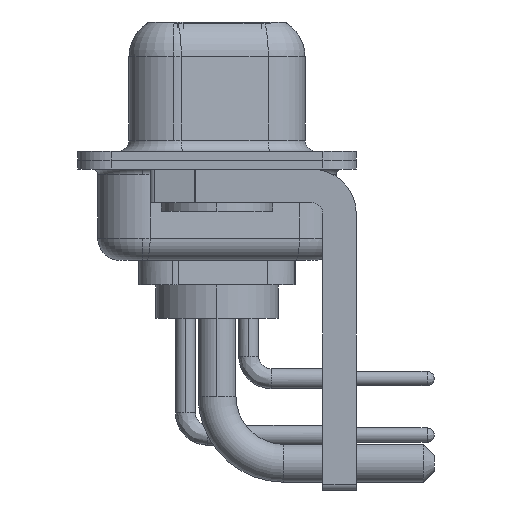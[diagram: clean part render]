
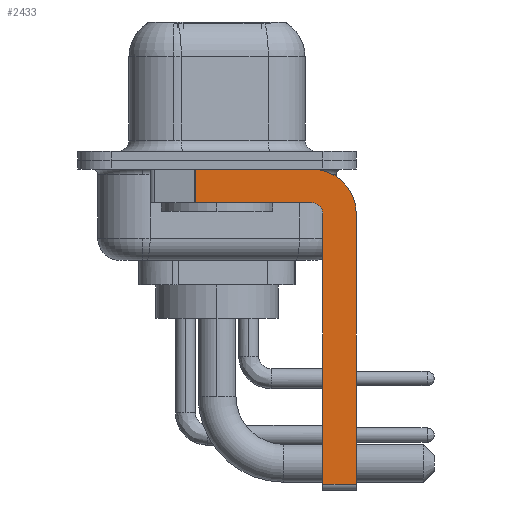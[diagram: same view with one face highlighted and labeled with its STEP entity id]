
A CAD part, left-side view. The second image highlights one B-rep face of the part: STEP entity #2433.
In plain terms, the highlighted planar face has unit normal (-1, 0, 0).
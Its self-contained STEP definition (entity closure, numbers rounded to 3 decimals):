
#480 = DIRECTION ( 'NONE',  ( 1., 0., 0. ) ) ;
#719 = CARTESIAN_POINT ( 'NONE',  ( -2.9, -4.25, -1.9 ) ) ;
#903 = AXIS2_PLACEMENT_3D ( 'NONE', #8533, #18773, #12303 ) ;
#1378 = VERTEX_POINT ( 'NONE', #12365 ) ;
#1528 = EDGE_CURVE ( 'NONE', #6450, #1378, #16380, .T. ) ;
#1864 = LINE ( 'NONE', #9912, #18777 ) ;
#2433 = ADVANCED_FACE ( 'NONE', ( #10746 ), #24308, .F. ) ;
#2564 = CARTESIAN_POINT ( 'NONE',  ( -2.9, -4.25, -14.55 ) ) ;
#2889 = CARTESIAN_POINT ( 'NONE',  ( -2.9, -4.75, -14.8 ) ) ;
#2917 = ORIENTED_EDGE ( 'NONE', *, *, #4839, .F. ) ;
#2998 = CIRCLE ( 'NONE', #21644, 0.5 ) ;
#3102 = CARTESIAN_POINT ( 'NONE',  ( -2.9, -4.75, -14.55 ) ) ;
#4381 = EDGE_CURVE ( 'NONE', #11176, #18284, #1864, .T. ) ;
#4839 = EDGE_CURVE ( 'NONE', #11176, #8308, #21286, .T. ) ;
#5808 = ORIENTED_EDGE ( 'NONE', *, *, #17295, .F. ) ;
#6160 = CARTESIAN_POINT ( 'NONE',  ( -2.9, -6.25, -2.4 ) ) ;
#6450 = VERTEX_POINT ( 'NONE', #3102 ) ;
#6570 = DIRECTION ( 'NONE',  ( 0., 0., -1. ) ) ;
#7180 = EDGE_CURVE ( 'NONE', #25567, #13903, #15662, .T. ) ;
#7836 = DIRECTION ( 'NONE',  ( 0., 0., -1. ) ) ;
#8308 = VERTEX_POINT ( 'NONE', #8537 ) ;
#8533 = CARTESIAN_POINT ( 'NONE',  ( -2.9, -4.25, -2.4 ) ) ;
#8537 = CARTESIAN_POINT ( 'NONE',  ( -2.9, -4.25, -0.4 ) ) ;
#8730 = ORIENTED_EDGE ( 'NONE', *, *, #25445, .F. ) ;
#8913 = CARTESIAN_POINT ( 'NONE',  ( -2.9, -6.25, -2.4 ) ) ;
#9010 = CARTESIAN_POINT ( 'NONE',  ( -2.9, -4.25, -2.4 ) ) ;
#9014 = VERTEX_POINT ( 'NONE', #21081 ) ;
#9421 = ORIENTED_EDGE ( 'NONE', *, *, #7180, .F. ) ;
#9679 = EDGE_LOOP ( 'NONE', ( #2917, #23237, #22040, #5808, #18373, #15643, #9421, #8730 ) ) ;
#9912 = CARTESIAN_POINT ( 'NONE',  ( -2.9, 0.978, -1.9 ) ) ;
#10204 = VECTOR ( 'NONE', #14741, 1000. ) ;
#10746 = FACE_OUTER_BOUND ( 'NONE', #9679, .T. ) ;
#10988 = VECTOR ( 'NONE', #24429, 1000. ) ;
#11068 = DIRECTION ( 'NONE',  ( 0., 0., 1. ) ) ;
#11176 = VERTEX_POINT ( 'NONE', #21080 ) ;
#11178 = DIRECTION ( 'NONE',  ( 0., -1., 0. ) ) ;
#12303 = DIRECTION ( 'NONE',  ( 0., 0., -1. ) ) ;
#12304 = CIRCLE ( 'NONE', #20184, 2. ) ;
#12365 = CARTESIAN_POINT ( 'NONE',  ( -2.9, -4.75, -2.4 ) ) ;
#12637 = DIRECTION ( 'NONE',  ( 0., 0., 1. ) ) ;
#13852 = VECTOR ( 'NONE', #11178, 1000. ) ;
#13903 = VERTEX_POINT ( 'NONE', #24674 ) ;
#14741 = DIRECTION ( 'NONE',  ( 0., 1., 0. ) ) ;
#15564 = CARTESIAN_POINT ( 'NONE',  ( -2.9, 0.978, -1.9 ) ) ;
#15643 = ORIENTED_EDGE ( 'NONE', *, *, #21193, .T. ) ;
#15662 = LINE ( 'NONE', #6160, #23373 ) ;
#16380 = LINE ( 'NONE', #2889, #19794 ) ;
#17158 = CARTESIAN_POINT ( 'NONE',  ( -2.9, 3., -0.4 ) ) ;
#17295 = EDGE_CURVE ( 'NONE', #1378, #9014, #2998, .T. ) ;
#18243 = CARTESIAN_POINT ( 'NONE',  ( -2.9, -4.25, -2.4 ) ) ;
#18284 = VERTEX_POINT ( 'NONE', #15564 ) ;
#18373 = ORIENTED_EDGE ( 'NONE', *, *, #1528, .F. ) ;
#18773 = DIRECTION ( 'NONE',  ( 1., 0., 0. ) ) ;
#18777 = VECTOR ( 'NONE', #7836, 1000. ) ;
#19794 = VECTOR ( 'NONE', #11068, 1000. ) ;
#20184 = AXIS2_PLACEMENT_3D ( 'NONE', #18243, #480, #6570 ) ;
#21080 = CARTESIAN_POINT ( 'NONE',  ( -2.9, 0.978, -0.4 ) ) ;
#21081 = CARTESIAN_POINT ( 'NONE',  ( -2.9, -4.25, -1.9 ) ) ;
#21193 = EDGE_CURVE ( 'NONE', #6450, #13903, #24686, .T. ) ;
#21286 = LINE ( 'NONE', #17158, #13852 ) ;
#21644 = AXIS2_PLACEMENT_3D ( 'NONE', #9010, #24514, #12637 ) ;
#21681 = EDGE_CURVE ( 'NONE', #9014, #18284, #24656, .T. ) ;
#22040 = ORIENTED_EDGE ( 'NONE', *, *, #21681, .F. ) ;
#23237 = ORIENTED_EDGE ( 'NONE', *, *, #4381, .T. ) ;
#23373 = VECTOR ( 'NONE', #23898, 1000. ) ;
#23898 = DIRECTION ( 'NONE',  ( 0., 0., -1. ) ) ;
#24308 = PLANE ( 'NONE',  #903 ) ;
#24429 = DIRECTION ( 'NONE',  ( 0., -1., 0. ) ) ;
#24514 = DIRECTION ( 'NONE',  ( -1., 0., 0. ) ) ;
#24656 = LINE ( 'NONE', #719, #10204 ) ;
#24674 = CARTESIAN_POINT ( 'NONE',  ( -2.9, -6.25, -14.55 ) ) ;
#24686 = LINE ( 'NONE', #2564, #10988 ) ;
#25445 = EDGE_CURVE ( 'NONE', #8308, #25567, #12304, .T. ) ;
#25567 = VERTEX_POINT ( 'NONE', #8913 ) ;
